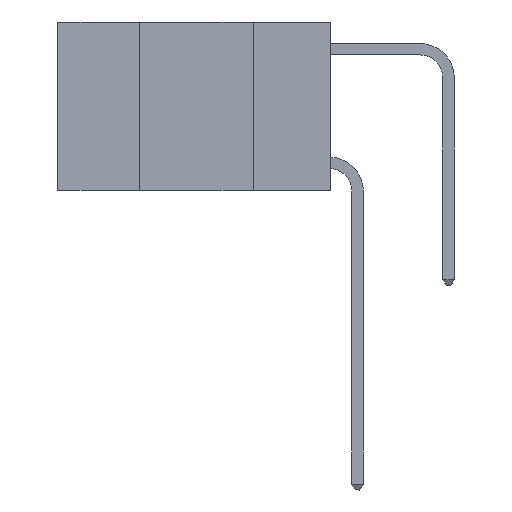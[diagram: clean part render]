
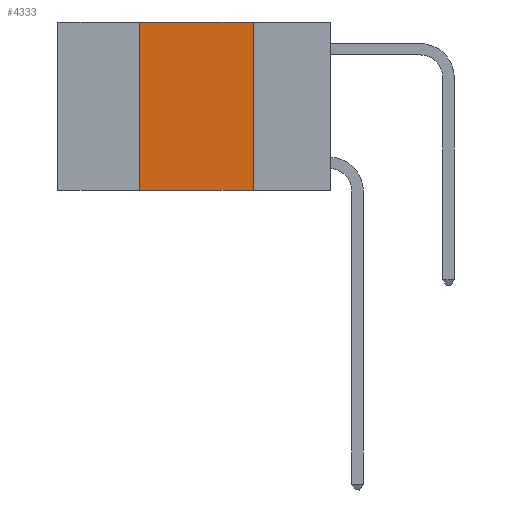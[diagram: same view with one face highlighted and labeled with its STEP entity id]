
A CAD part, left-side view. The second image highlights one B-rep face of the part: STEP entity #4333.
In plain terms, the highlighted planar face has unit normal (-1, 0, 0).
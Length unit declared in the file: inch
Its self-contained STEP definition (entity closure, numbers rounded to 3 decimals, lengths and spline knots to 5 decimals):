
#373 = AXIS2_PLACEMENT_3D ( 'NONE', #23158, #4572, #17750 ) ;
#1081 = LINE ( 'NONE', #23723, #11236 ) ;
#1768 = DIRECTION ( 'NONE',  ( 0., 0., -1. ) ) ;
#2292 = VECTOR ( 'NONE', #1768, 39.37008 ) ;
#2617 = DIRECTION ( 'NONE',  ( 0., -1., 0. ) ) ;
#2637 = PLANE ( 'NONE',  #373 ) ;
#2896 = EDGE_LOOP ( 'NONE', ( #13283, #18171, #23570, #4328 ) ) ;
#4328 = ORIENTED_EDGE ( 'NONE', *, *, #19598, .T. ) ;
#4333 = ADVANCED_FACE ( 'NONE', ( #19863 ), #2637, .F. ) ;
#4572 = DIRECTION ( 'NONE',  ( 1., 0., 0. ) ) ;
#6351 = CARTESIAN_POINT ( 'NONE',  ( 0., 0.42, 0. ) ) ;
#7212 = VERTEX_POINT ( 'NONE', #10131 ) ;
#8316 = CARTESIAN_POINT ( 'NONE',  ( 0., 0.6, -0.37 ) ) ;
#8597 = LINE ( 'NONE', #17217, #17969 ) ;
#9611 = CARTESIAN_POINT ( 'NONE',  ( 0., 0.42, -0.37 ) ) ;
#10131 = CARTESIAN_POINT ( 'NONE',  ( 0., 0.17, -0.37 ) ) ;
#10280 = EDGE_CURVE ( 'NONE', #10684, #23102, #1081, .T. ) ;
#10684 = VERTEX_POINT ( 'NONE', #6351 ) ;
#11236 = VECTOR ( 'NONE', #16529, 39.37008 ) ;
#13283 = ORIENTED_EDGE ( 'NONE', *, *, #22028, .F. ) ;
#13444 = VERTEX_POINT ( 'NONE', #9611 ) ;
#13985 = VECTOR ( 'NONE', #2617, 39.37008 ) ;
#15170 = LINE ( 'NONE', #8316, #13985 ) ;
#16529 = DIRECTION ( 'NONE',  ( 0., -1., 0. ) ) ;
#17217 = CARTESIAN_POINT ( 'NONE',  ( 0., 0.42, 0. ) ) ;
#17750 = DIRECTION ( 'NONE',  ( 0., 0., -1. ) ) ;
#17969 = VECTOR ( 'NONE', #19035, 39.37008 ) ;
#18171 = ORIENTED_EDGE ( 'NONE', *, *, #10280, .F. ) ;
#19035 = DIRECTION ( 'NONE',  ( 0., 0., 1. ) ) ;
#19598 = EDGE_CURVE ( 'NONE', #13444, #7212, #15170, .T. ) ;
#19863 = FACE_OUTER_BOUND ( 'NONE', #2896, .T. ) ;
#20833 = EDGE_CURVE ( 'NONE', #13444, #10684, #8597, .T. ) ;
#21887 = CARTESIAN_POINT ( 'NONE',  ( 0., 0.17, 0. ) ) ;
#22028 = EDGE_CURVE ( 'NONE', #23102, #7212, #22230, .T. ) ;
#22230 = LINE ( 'NONE', #24128, #2292 ) ;
#23102 = VERTEX_POINT ( 'NONE', #21887 ) ;
#23158 = CARTESIAN_POINT ( 'NONE',  ( 0., 0.6, 0. ) ) ;
#23570 = ORIENTED_EDGE ( 'NONE', *, *, #20833, .F. ) ;
#23723 = CARTESIAN_POINT ( 'NONE',  ( 0., 0.6, 0. ) ) ;
#24128 = CARTESIAN_POINT ( 'NONE',  ( 0., 0.17, 0. ) ) ;
